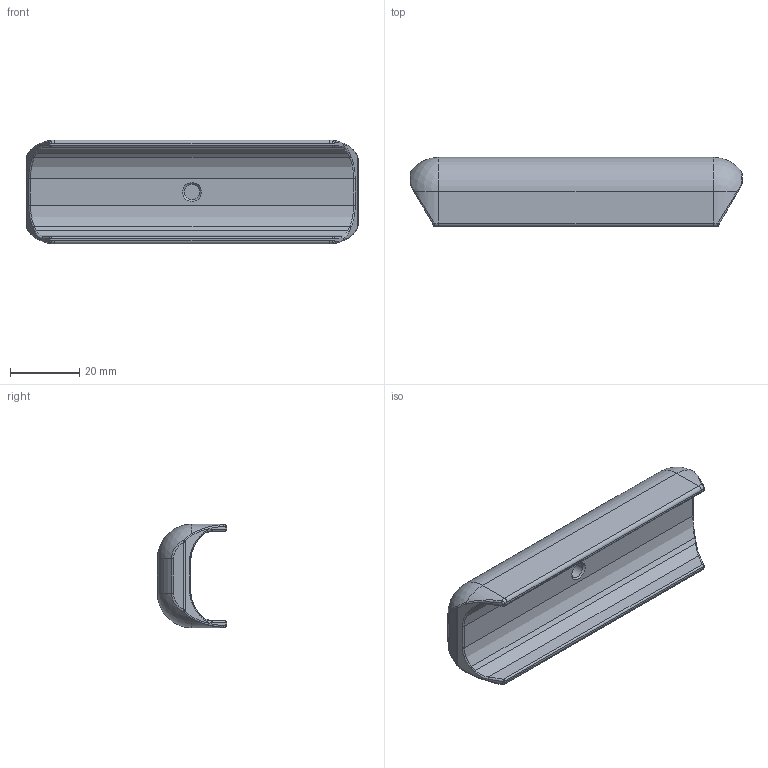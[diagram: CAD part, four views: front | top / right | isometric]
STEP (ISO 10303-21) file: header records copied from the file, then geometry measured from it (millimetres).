
FILE_DESCRIPTION (( 'STEP AP203' ), '1' );
FILE_NAME ('MOD9_G36_stock_cheek-rest.STEP', '2020-07-07T01:46:03', ( '' ), ( '' ), 'SwSTEP 2.0', 'SolidWorks 2016', '' );
FILE_SCHEMA (( 'CONFIG_CONTROL_DESIGN' ));
Length unit declared in the file: millimetre
Products named in the file (1): MOD9_G36_stock_cheek-rest
Bounding box: 96 x 20 x 30 mm (x, y, z)
Volume: 28456.7 mm3; surface area: 10003.9 mm2
Topology: 1 solids, 1 shells, 95 faces, 211 edges, 115 vertices
Faces by surface type: cylinder 31, bspline 28, plane 15, torus 12, sphere 8, cone 1
Full cylindrical faces by diameter (mm): 4.5 x1
Entity records: 3375 total; most frequent: CARTESIAN_POINT 1456, ORIENTED_EDGE 410, DIRECTION 324, EDGE_CURVE 205, AXIS2_PLACEMENT_3D 131, VERTEX_POINT 115, EDGE_LOOP 98, FACE_OUTER_BOUND 96
